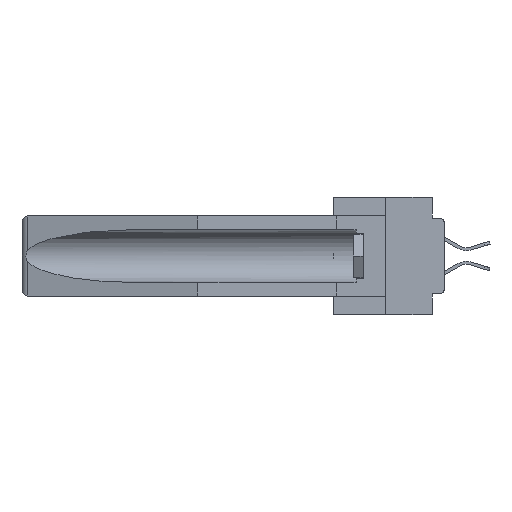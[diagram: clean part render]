
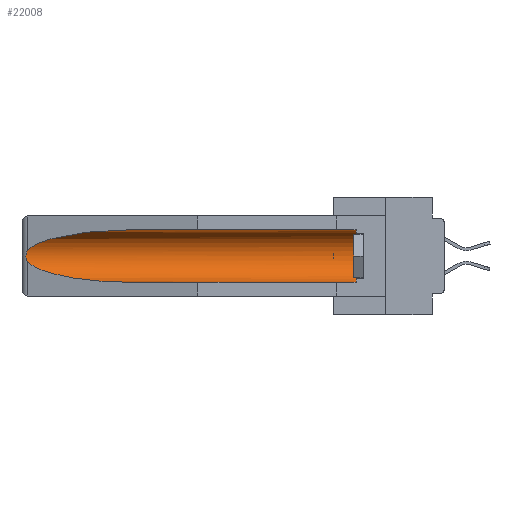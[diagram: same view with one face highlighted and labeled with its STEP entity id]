
A CAD part, left-side view. The second image highlights one B-rep face of the part: STEP entity #22008.
In plain terms, the highlighted cylindrical face has radius 2.857 mm (diameter 5.715 mm), a partial arc.
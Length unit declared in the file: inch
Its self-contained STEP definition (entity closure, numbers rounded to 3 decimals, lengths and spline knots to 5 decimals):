
#621 = CARTESIAN_POINT ( 'NONE',  ( 0.26537, 1.52718, -0.14972 ) ) ;
#1141 = DIRECTION ( 'NONE',  ( 0., 0., 1. ) ) ;
#1342 = CARTESIAN_POINT ( 'NONE',  ( 0.155, 0.126, -0.1715 ) ) ;
#1393 = B_SPLINE_CURVE_WITH_KNOTS ( 'NONE', 3,
 ( #2767, #6077, #18625, #24831, #31202, #12254, #21122, #27295, #39862, #15136 ),
 .UNSPECIFIED., .F., .F.,
 ( 4, 2, 2, 2, 4 ),
 ( 0., 0.00029, 0.00058, 0.00087, 0.00117 ),
 .UNSPECIFIED. ) ;
#1663 = EDGE_CURVE ( 'NONE', #28994, #27548, #31219, .T. ) ;
#2189 = CARTESIAN_POINT ( 'NONE',  ( 0.155, 1.07973, -0.059 ) ) ;
#2767 = CARTESIAN_POINT ( 'NONE',  ( 0.26537, 1.52718, -0.14972 ) ) ;
#5131 =( BOUNDED_CURVE ( )  B_SPLINE_CURVE ( 3, ( #33669, #18605, #27693, #17992 ),
 .UNSPECIFIED., .F., .F. ) 
 B_SPLINE_CURVE_WITH_KNOTS ( ( 4, 4 ),
 ( 0.1948, 1.5708 ),
 .UNSPECIFIED. ) 
 CURVE ( )  GEOMETRIC_REPRESENTATION_ITEM ( )  RATIONAL_B_SPLINE_CURVE ( ( 1., 0.848, 0.848, 1. ) ) 
 REPRESENTATION_ITEM ( '' )  );
#5285 = ORIENTED_EDGE ( 'NONE', *, *, #1663, .T. ) ;
#5323 = EDGE_CURVE ( 'NONE', #19878, #5956, #1393, .T. ) ;
#5956 = VERTEX_POINT ( 'NONE', #9512 ) ;
#6077 = CARTESIAN_POINT ( 'NONE',  ( 0.26597, 1.52961, -0.15275 ) ) ;
#6944 = CARTESIAN_POINT ( 'NONE',  ( 0.155, 1.07973, -0.284 ) ) ;
#7015 = CARTESIAN_POINT ( 'NONE',  ( 0.155, -0.30754, -0.284 ) ) ;
#7029 = VECTOR ( 'NONE', #8172, 39.37008 ) ;
#7332 = EDGE_CURVE ( 'NONE', #25198, #19878, #32800, .T. ) ;
#8172 = DIRECTION ( 'NONE',  ( 0., 1., 0. ) ) ;
#9512 = CARTESIAN_POINT ( 'NONE',  ( 0.26537, 1.52718, -0.19328 ) ) ;
#10108 = LINE ( 'NONE', #7015, #7029 ) ;
#10965 = ORIENTED_EDGE ( 'NONE', *, *, #30517, .T. ) ;
#11892 = FACE_OUTER_BOUND ( 'NONE', #35542, .T. ) ;
#12254 = CARTESIAN_POINT ( 'NONE',  ( 0.2675, 1.53308, -0.17534 ) ) ;
#15118 = ORIENTED_EDGE ( 'NONE', *, *, #5323, .T. ) ;
#15136 = CARTESIAN_POINT ( 'NONE',  ( 0.26537, 1.52718, -0.19328 ) ) ;
#16911 = VECTOR ( 'NONE', #36381, 39.37008 ) ;
#17992 = CARTESIAN_POINT ( 'NONE',  ( 0.155, 1.07973, -0.284 ) ) ;
#18048 = CARTESIAN_POINT ( 'NONE',  ( 0.155, -0.30754, -0.1715 ) ) ;
#18605 = CARTESIAN_POINT ( 'NONE',  ( 0.25451, 1.48313, -0.24835 ) ) ;
#18625 = CARTESIAN_POINT ( 'NONE',  ( 0.26654, 1.53092, -0.15636 ) ) ;
#19451 = CARTESIAN_POINT ( 'NONE',  ( 0.155, 0.126, -0.059 ) ) ;
#19464 = AXIS2_PLACEMENT_3D ( 'NONE', #18048, #27332, #30234 ) ;
#19878 = VERTEX_POINT ( 'NONE', #621 ) ;
#21122 = CARTESIAN_POINT ( 'NONE',  ( 0.2673, 1.53269, -0.17917 ) ) ;
#21711 = VERTEX_POINT ( 'NONE', #6944 ) ;
#22008 = ADVANCED_FACE ( 'NONE', ( #11892 ), #24864, .F. ) ;
#22861 = EDGE_CURVE ( 'NONE', #28994, #21711, #10108, .T. ) ;
#23834 = LINE ( 'NONE', #30228, #16911 ) ;
#24381 = EDGE_CURVE ( 'NONE', #5956, #21711, #5131, .T. ) ;
#24831 = CARTESIAN_POINT ( 'NONE',  ( 0.2673, 1.5327, -0.16383 ) ) ;
#24864 = CYLINDRICAL_SURFACE ( 'NONE', #19464, 0.1125 ) ;
#25198 = VERTEX_POINT ( 'NONE', #2189 ) ;
#25597 = ORIENTED_EDGE ( 'NONE', *, *, #24381, .T. ) ;
#26504 = CARTESIAN_POINT ( 'NONE',  ( 0.155, 0.126, -0.284 ) ) ;
#27295 = CARTESIAN_POINT ( 'NONE',  ( 0.26655, 1.53094, -0.18657 ) ) ;
#27332 = DIRECTION ( 'NONE',  ( 0., 1., 0. ) ) ;
#27548 = VERTEX_POINT ( 'NONE', #19451 ) ;
#27647 = ORIENTED_EDGE ( 'NONE', *, *, #22861, .F. ) ;
#27693 = CARTESIAN_POINT ( 'NONE',  ( 0.21114, 1.30732, -0.284 ) ) ;
#27710 = CARTESIAN_POINT ( 'NONE',  ( 0.26537, 1.52718, -0.14972 ) ) ;
#28994 = VERTEX_POINT ( 'NONE', #26504 ) ;
#29239 = AXIS2_PLACEMENT_3D ( 'NONE', #1342, #29766, #1141 ) ;
#29766 = DIRECTION ( 'NONE',  ( 0., -1., 0. ) ) ;
#30228 = CARTESIAN_POINT ( 'NONE',  ( 0.155, -0.30754, -0.059 ) ) ;
#30234 = DIRECTION ( 'NONE',  ( 0., 0., 1. ) ) ;
#30517 = EDGE_CURVE ( 'NONE', #27548, #25198, #23834, .T. ) ;
#31202 = CARTESIAN_POINT ( 'NONE',  ( 0.2675, 1.53308, -0.16763 ) ) ;
#31219 = CIRCLE ( 'NONE', #29239, 0.1125 ) ;
#31619 = CARTESIAN_POINT ( 'NONE',  ( 0.155, 1.07973, -0.059 ) ) ;
#32800 =( BOUNDED_CURVE ( )  B_SPLINE_CURVE ( 3, ( #31619, #37389, #34297, #27710 ),
 .UNSPECIFIED., .F., .F. ) 
 B_SPLINE_CURVE_WITH_KNOTS ( ( 4, 4 ),
 ( 4.71239, 6.08839 ),
 .UNSPECIFIED. ) 
 CURVE ( )  GEOMETRIC_REPRESENTATION_ITEM ( )  RATIONAL_B_SPLINE_CURVE ( ( 1., 0.848, 0.848, 1. ) ) 
 REPRESENTATION_ITEM ( '' )  );
#33669 = CARTESIAN_POINT ( 'NONE',  ( 0.26537, 1.52718, -0.19328 ) ) ;
#34297 = CARTESIAN_POINT ( 'NONE',  ( 0.25451, 1.48313, -0.09465 ) ) ;
#35542 = EDGE_LOOP ( 'NONE', ( #36814, #15118, #25597, #27647, #5285, #10965 ) ) ;
#36381 = DIRECTION ( 'NONE',  ( 0., 1., 0. ) ) ;
#36814 = ORIENTED_EDGE ( 'NONE', *, *, #7332, .T. ) ;
#37389 = CARTESIAN_POINT ( 'NONE',  ( 0.21114, 1.30732, -0.059 ) ) ;
#39862 = CARTESIAN_POINT ( 'NONE',  ( 0.26597, 1.5296, -0.19026 ) ) ;
